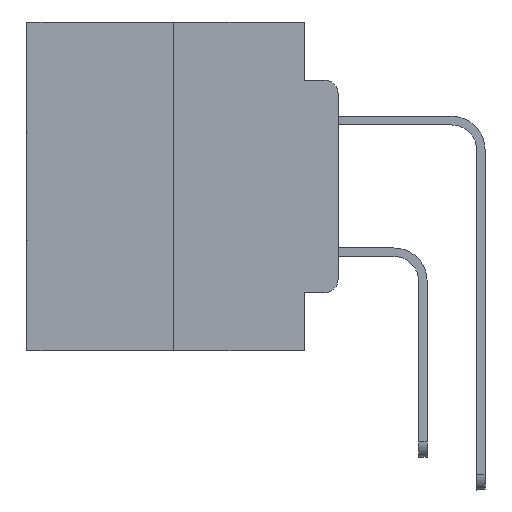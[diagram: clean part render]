
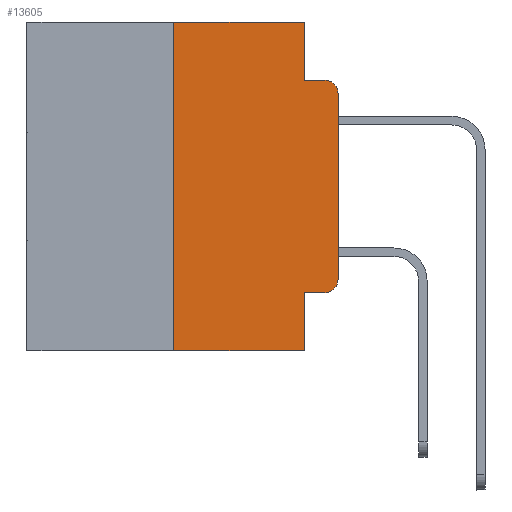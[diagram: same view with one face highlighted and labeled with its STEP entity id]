
A CAD part, left-side view. The second image highlights one B-rep face of the part: STEP entity #13605.
In plain terms, the highlighted planar face has unit normal (-1, 0, 0).
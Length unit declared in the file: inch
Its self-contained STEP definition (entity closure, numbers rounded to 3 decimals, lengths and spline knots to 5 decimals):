
#794 = DIRECTION ( 'NONE',  ( 0., -1., 0. ) ) ;
#1252 = CARTESIAN_POINT ( 'NONE',  ( 0., 0.25, 0. ) ) ;
#1299 = DIRECTION ( 'NONE',  ( -1., 0., 0. ) ) ;
#2181 = ORIENTED_EDGE ( 'NONE', *, *, #11970, .F. ) ;
#2748 = EDGE_LOOP ( 'NONE', ( #3983, #22975, #11613, #23686, #7584, #2181, #21276, #3650, #23340, #24066 ) ) ;
#2788 = DIRECTION ( 'NONE',  ( 0., 0., -1. ) ) ;
#2922 = FACE_OUTER_BOUND ( 'NONE', #2748, .T. ) ;
#2973 = AXIS2_PLACEMENT_3D ( 'NONE', #6952, #25232, #11666 ) ;
#3048 = VERTEX_POINT ( 'NONE', #27551 ) ;
#3366 = CIRCLE ( 'NONE', #25749, 0.02 ) ;
#3589 = CARTESIAN_POINT ( 'NONE',  ( 0., 0.051, -0.0885 ) ) ;
#3650 = ORIENTED_EDGE ( 'NONE', *, *, #10415, .F. ) ;
#3983 = ORIENTED_EDGE ( 'NONE', *, *, #21154, .T. ) ;
#4321 = LINE ( 'NONE', #6619, #10518 ) ;
#4615 = VERTEX_POINT ( 'NONE', #20054 ) ;
#5722 = EDGE_CURVE ( 'NONE', #21663, #27717, #26095, .T. ) ;
#5913 = VECTOR ( 'NONE', #794, 39.37008 ) ;
#6235 = CARTESIAN_POINT ( 'NONE',  ( 0., 0.051, -0.0885 ) ) ;
#6619 = CARTESIAN_POINT ( 'NONE',  ( 0., 0., 0. ) ) ;
#6620 = CARTESIAN_POINT ( 'NONE',  ( 0., 0.051, 0. ) ) ;
#6656 = CARTESIAN_POINT ( 'NONE',  ( 0., 0., -0.3915 ) ) ;
#6939 = CARTESIAN_POINT ( 'NONE',  ( 0., 0.051, -0.5 ) ) ;
#6952 = CARTESIAN_POINT ( 'NONE',  ( 0., 0.473, 0. ) ) ;
#7458 = DIRECTION ( 'NONE',  ( 0., 0., -1. ) ) ;
#7584 = ORIENTED_EDGE ( 'NONE', *, *, #20432, .F. ) ;
#7745 = VECTOR ( 'NONE', #17688, 39.37008 ) ;
#8097 = VERTEX_POINT ( 'NONE', #28114 ) ;
#8110 = DIRECTION ( 'NONE',  ( -1., 0., 0. ) ) ;
#8157 = DIRECTION ( 'NONE',  ( 0., -1., 0. ) ) ;
#8830 = EDGE_CURVE ( 'NONE', #3048, #21663, #13559, .T. ) ;
#9040 = LINE ( 'NONE', #27061, #20563 ) ;
#9215 = EDGE_CURVE ( 'NONE', #20417, #27846, #20330, .T. ) ;
#10415 = EDGE_CURVE ( 'NONE', #3048, #27846, #16021, .T. ) ;
#10518 = VECTOR ( 'NONE', #22648, 39.37008 ) ;
#11613 = ORIENTED_EDGE ( 'NONE', *, *, #16621, .F. ) ;
#11666 = DIRECTION ( 'NONE',  ( 0., 0., -1. ) ) ;
#11970 = EDGE_CURVE ( 'NONE', #20417, #20765, #9040, .T. ) ;
#12701 = CARTESIAN_POINT ( 'NONE',  ( 0., 0.473, -0.5 ) ) ;
#13559 = LINE ( 'NONE', #23687, #5913 ) ;
#13605 = ADVANCED_FACE ( 'NONE', ( #2922 ), #22976, .F. ) ;
#15044 = DIRECTION ( 'NONE',  ( 0., -1., 0. ) ) ;
#15097 = EDGE_CURVE ( 'NONE', #28346, #19444, #19070, .T. ) ;
#15244 = CARTESIAN_POINT ( 'NONE',  ( 0., 0.02, -0.1085 ) ) ;
#16021 = LINE ( 'NONE', #24120, #25119 ) ;
#16311 = CARTESIAN_POINT ( 'NONE',  ( 0., 0.473, 0. ) ) ;
#16621 = EDGE_CURVE ( 'NONE', #19444, #8097, #20744, .T. ) ;
#17528 = DIRECTION ( 'NONE',  ( 0., 0., -1. ) ) ;
#17688 = DIRECTION ( 'NONE',  ( 0., -1., 0. ) ) ;
#17818 = CARTESIAN_POINT ( 'NONE',  ( 0., 0.02, -0.3915 ) ) ;
#18093 = AXIS2_PLACEMENT_3D ( 'NONE', #17818, #8110, #7458 ) ;
#18129 = EDGE_CURVE ( 'NONE', #4615, #8097, #3366, .T. ) ;
#18930 = CARTESIAN_POINT ( 'NONE',  ( 0., 0.051, 0. ) ) ;
#19070 = LINE ( 'NONE', #18930, #29496 ) ;
#19444 = VERTEX_POINT ( 'NONE', #3589 ) ;
#19539 = DIRECTION ( 'NONE',  ( 0., 0., -1. ) ) ;
#20054 = CARTESIAN_POINT ( 'NONE',  ( 0., 0., -0.1085 ) ) ;
#20330 = LINE ( 'NONE', #12701, #26243 ) ;
#20348 = DIRECTION ( 'NONE',  ( 0., 0., 1. ) ) ;
#20417 = VERTEX_POINT ( 'NONE', #27450 ) ;
#20432 = EDGE_CURVE ( 'NONE', #20765, #28346, #24725, .T. ) ;
#20563 = VECTOR ( 'NONE', #20348, 39.37008 ) ;
#20744 = LINE ( 'NONE', #6235, #7745 ) ;
#20765 = VERTEX_POINT ( 'NONE', #1252 ) ;
#21154 = EDGE_CURVE ( 'NONE', #27717, #4615, #4321, .T. ) ;
#21276 = ORIENTED_EDGE ( 'NONE', *, *, #9215, .T. ) ;
#21663 = VERTEX_POINT ( 'NONE', #22238 ) ;
#22238 = CARTESIAN_POINT ( 'NONE',  ( 0., 0.02, -0.4115 ) ) ;
#22648 = DIRECTION ( 'NONE',  ( 0., 0., 1. ) ) ;
#22975 = ORIENTED_EDGE ( 'NONE', *, *, #18129, .T. ) ;
#22976 = PLANE ( 'NONE',  #2973 ) ;
#23340 = ORIENTED_EDGE ( 'NONE', *, *, #8830, .T. ) ;
#23686 = ORIENTED_EDGE ( 'NONE', *, *, #15097, .F. ) ;
#23687 = CARTESIAN_POINT ( 'NONE',  ( 0., 0.051, -0.4115 ) ) ;
#24027 = VECTOR ( 'NONE', #8157, 39.37008 ) ;
#24066 = ORIENTED_EDGE ( 'NONE', *, *, #5722, .T. ) ;
#24120 = CARTESIAN_POINT ( 'NONE',  ( 0., 0.051, 0. ) ) ;
#24725 = LINE ( 'NONE', #16311, #24027 ) ;
#25119 = VECTOR ( 'NONE', #19539, 39.37008 ) ;
#25232 = DIRECTION ( 'NONE',  ( 1., 0., 0. ) ) ;
#25749 = AXIS2_PLACEMENT_3D ( 'NONE', #15244, #1299, #17528 ) ;
#26095 = CIRCLE ( 'NONE', #18093, 0.02 ) ;
#26243 = VECTOR ( 'NONE', #15044, 39.37008 ) ;
#27061 = CARTESIAN_POINT ( 'NONE',  ( 0., 0.25, 0. ) ) ;
#27450 = CARTESIAN_POINT ( 'NONE',  ( 0., 0.25, -0.5 ) ) ;
#27551 = CARTESIAN_POINT ( 'NONE',  ( 0., 0.051, -0.4115 ) ) ;
#27717 = VERTEX_POINT ( 'NONE', #6656 ) ;
#27846 = VERTEX_POINT ( 'NONE', #6939 ) ;
#28114 = CARTESIAN_POINT ( 'NONE',  ( 0., 0.02, -0.0885 ) ) ;
#28346 = VERTEX_POINT ( 'NONE', #6620 ) ;
#29496 = VECTOR ( 'NONE', #2788, 39.37008 ) ;
